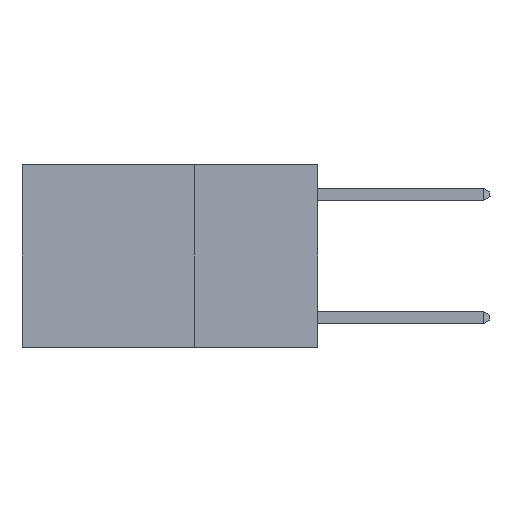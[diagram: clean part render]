
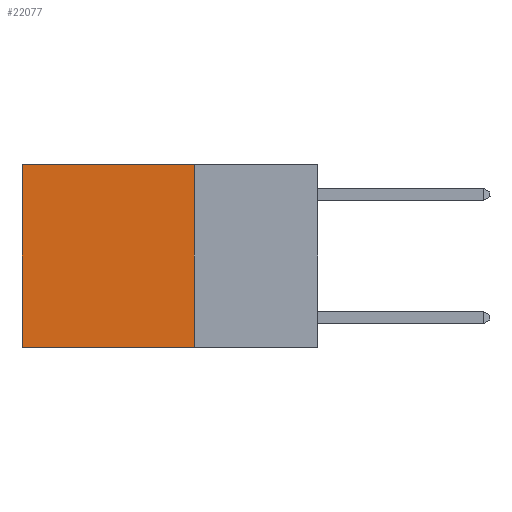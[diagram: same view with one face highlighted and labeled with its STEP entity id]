
A CAD part, left-side view. The second image highlights one B-rep face of the part: STEP entity #22077.
In plain terms, the highlighted planar face has unit normal (-1, 0, 0).
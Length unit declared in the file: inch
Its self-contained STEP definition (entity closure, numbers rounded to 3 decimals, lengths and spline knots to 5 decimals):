
#1636 = DIRECTION ( 'NONE',  ( 0., 0., -1. ) ) ;
#1655 = CARTESIAN_POINT ( 'NONE',  ( 0.2625, 0.6, 0. ) ) ;
#1866 = CARTESIAN_POINT ( 'NONE',  ( 0.2625, 0.25, 0. ) ) ;
#2292 = VECTOR ( 'NONE', #1636, 39.37008 ) ;
#3080 = VECTOR ( 'NONE', #17853, 39.37008 ) ;
#3154 = CARTESIAN_POINT ( 'NONE',  ( 0.2625, 0.25, -0.37 ) ) ;
#4205 = EDGE_CURVE ( 'NONE', #10396, #13495, #9900, .T. ) ;
#4217 = DIRECTION ( 'NONE',  ( 0., 0., -1. ) ) ;
#6618 = CARTESIAN_POINT ( 'NONE',  ( 0.2625, 0.6, 0. ) ) ;
#8455 = CARTESIAN_POINT ( 'NONE',  ( 0.2625, 0.25, -0.37 ) ) ;
#9210 = LINE ( 'NONE', #10869, #2292 ) ;
#9464 = EDGE_CURVE ( 'NONE', #10087, #13495, #14638, .T. ) ;
#9900 = LINE ( 'NONE', #8455, #26943 ) ;
#9982 = EDGE_CURVE ( 'NONE', #17824, #10396, #9210, .T. ) ;
#10087 = VERTEX_POINT ( 'NONE', #6618 ) ;
#10396 = VERTEX_POINT ( 'NONE', #3154 ) ;
#10630 = VECTOR ( 'NONE', #12769, 39.37008 ) ;
#10869 = CARTESIAN_POINT ( 'NONE',  ( 0.2625, 0.25, 0. ) ) ;
#11098 = PLANE ( 'NONE',  #12554 ) ;
#11462 = ORIENTED_EDGE ( 'NONE', *, *, #25185, .T. ) ;
#11954 = ORIENTED_EDGE ( 'NONE', *, *, #9464, .T. ) ;
#12554 = AXIS2_PLACEMENT_3D ( 'NONE', #1866, #18072, #4217 ) ;
#12769 = DIRECTION ( 'NONE',  ( 0., 1., 0. ) ) ;
#13495 = VERTEX_POINT ( 'NONE', #15450 ) ;
#14638 = LINE ( 'NONE', #1655, #3080 ) ;
#15375 = DIRECTION ( 'NONE',  ( 0., 1., 0. ) ) ;
#15444 = ORIENTED_EDGE ( 'NONE', *, *, #4205, .F. ) ;
#15450 = CARTESIAN_POINT ( 'NONE',  ( 0.2625, 0.6, -0.37 ) ) ;
#16077 = ORIENTED_EDGE ( 'NONE', *, *, #9982, .F. ) ;
#16767 = LINE ( 'NONE', #24215, #10630 ) ;
#17824 = VERTEX_POINT ( 'NONE', #18788 ) ;
#17853 = DIRECTION ( 'NONE',  ( 0., 0., -1. ) ) ;
#18072 = DIRECTION ( 'NONE',  ( 1., 0., 0. ) ) ;
#18788 = CARTESIAN_POINT ( 'NONE',  ( 0.2625, 0.25, 0. ) ) ;
#22077 = ADVANCED_FACE ( 'NONE', ( #28522 ), #11098, .F. ) ;
#23565 = EDGE_LOOP ( 'NONE', ( #11954, #15444, #16077, #11462 ) ) ;
#24215 = CARTESIAN_POINT ( 'NONE',  ( 0.2625, 0.25, 0. ) ) ;
#25185 = EDGE_CURVE ( 'NONE', #17824, #10087, #16767, .T. ) ;
#26943 = VECTOR ( 'NONE', #15375, 39.37008 ) ;
#28522 = FACE_OUTER_BOUND ( 'NONE', #23565, .T. ) ;
